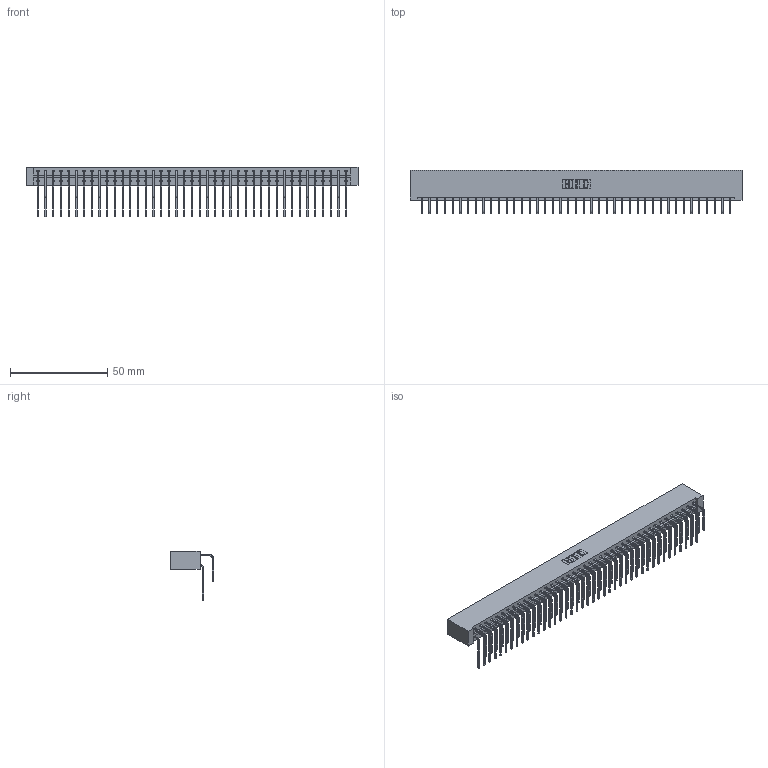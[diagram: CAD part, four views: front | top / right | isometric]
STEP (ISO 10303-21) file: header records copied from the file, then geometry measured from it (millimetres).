
FILE_DESCRIPTION (( 'STEP AP203' ), '1' );
FILE_NAME ('833-082-558-201.STEP', '2020-06-06T00:17:42', ( '' ), ( '' ), 'SwSTEP 2.0', 'SolidWorks 2020', '' );
FILE_SCHEMA (( 'CONFIG_CONTROL_DESIGN' ));
Length unit declared in the file: inch
Products named in the file (4): 345-292-001_558 559 Tail - 1; 345-292-001_558 Tail - 2; 833-082-558-201; 833 Part_Lugless
Assembly tree (83 placements, depth 2):
  833-082-558-201
    833 Part_Lugless
    345-292-001_558 559 Tail - 1  x41
    345-292-001_558 Tail - 2  x41
Bounding box: 170.71 x 22.17 x 25.53 mm (x, y, z)
Volume: 18524.8 mm3; surface area: 24270.7 mm2
Topology: 83 solids, 83 shells, 4534 faces, 13489 edges, 8882 vertices
Faces by surface type: plane 3182, cylinder 1352
Entity records: 28013 total; most frequent: CARTESIAN_POINT 4693, ORIENTED_EDGE 4578, DIRECTION 3985, EDGE_CURVE 2289, VECTOR 2129, LINE 2129, VERTEX_POINT 1522, AXIS2_PLACEMENT_3D 928
